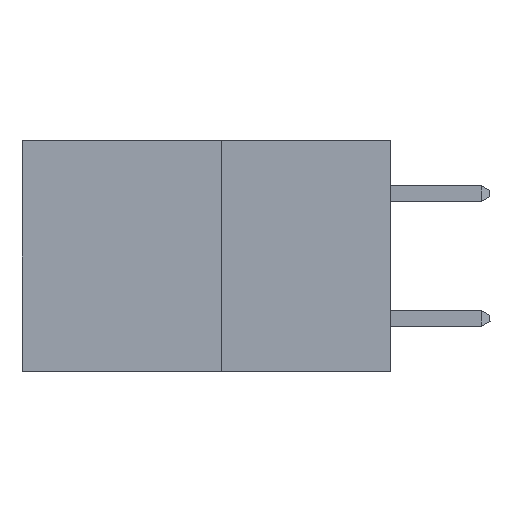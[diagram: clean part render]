
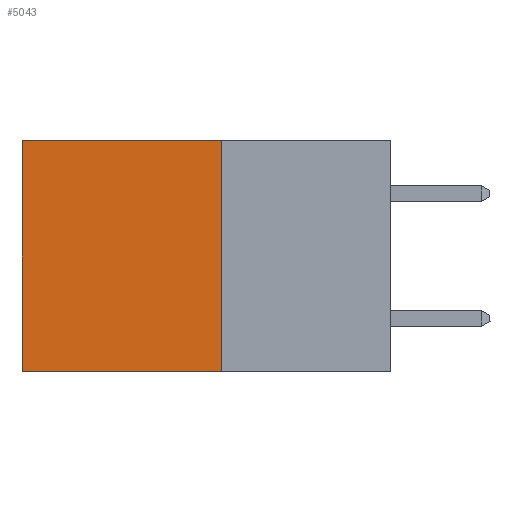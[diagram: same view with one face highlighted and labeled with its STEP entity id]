
A CAD part, left-side view. The second image highlights one B-rep face of the part: STEP entity #5043.
In plain terms, the highlighted planar face has unit normal (-1, 0, 0).
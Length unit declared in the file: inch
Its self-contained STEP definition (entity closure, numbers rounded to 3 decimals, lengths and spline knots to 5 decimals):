
#321 = AXIS2_PLACEMENT_3D ( 'NONE', #8548, #8375, #8352 ) ;
#361 = CARTESIAN_POINT ( 'NONE',  ( 0.277, 0.27, 0. ) ) ;
#3229 = DIRECTION ( 'NONE',  ( 0., 0., -1. ) ) ;
#4635 = VECTOR ( 'NONE', #23916, 39.37008 ) ;
#4870 = EDGE_CURVE ( 'NONE', #6382, #26060, #16829, .T. ) ;
#5043 = ADVANCED_FACE ( 'NONE', ( #12200 ), #8819, .F. ) ;
#5691 = CARTESIAN_POINT ( 'NONE',  ( 0.277, 0.27, 0. ) ) ;
#6382 = VERTEX_POINT ( 'NONE', #19928 ) ;
#6385 = CARTESIAN_POINT ( 'NONE',  ( 0.277, 0.59, 0. ) ) ;
#7436 = ORIENTED_EDGE ( 'NONE', *, *, #4870, .F. ) ;
#7509 = EDGE_CURVE ( 'NONE', #14707, #26060, #19439, .T. ) ;
#7871 = VERTEX_POINT ( 'NONE', #5691 ) ;
#8352 = DIRECTION ( 'NONE',  ( 0., 0., -1. ) ) ;
#8375 = DIRECTION ( 'NONE',  ( 1., 0., 0. ) ) ;
#8548 = CARTESIAN_POINT ( 'NONE',  ( 0.277, 0.27, -0.37 ) ) ;
#8819 = PLANE ( 'NONE',  #321 ) ;
#9080 = DIRECTION ( 'NONE',  ( 0., 0., -1. ) ) ;
#9460 = LINE ( 'NONE', #16090, #26317 ) ;
#11034 = ORIENTED_EDGE ( 'NONE', *, *, #15144, .F. ) ;
#11118 = LINE ( 'NONE', #361, #4635 ) ;
#11879 = VECTOR ( 'NONE', #12729, 39.37008 ) ;
#12200 = FACE_OUTER_BOUND ( 'NONE', #14894, .T. ) ;
#12729 = DIRECTION ( 'NONE',  ( 0., 1., 0. ) ) ;
#12757 = CARTESIAN_POINT ( 'NONE',  ( 0.277, 0.27, -0.37 ) ) ;
#13792 = VECTOR ( 'NONE', #9080, 39.37008 ) ;
#14707 = VERTEX_POINT ( 'NONE', #6385 ) ;
#14894 = EDGE_LOOP ( 'NONE', ( #15202, #7436, #11034, #25465 ) ) ;
#15144 = EDGE_CURVE ( 'NONE', #7871, #6382, #9460, .T. ) ;
#15202 = ORIENTED_EDGE ( 'NONE', *, *, #7509, .T. ) ;
#16090 = CARTESIAN_POINT ( 'NONE',  ( 0.277, 0.27, -0.37 ) ) ;
#16829 = LINE ( 'NONE', #12757, #11879 ) ;
#18511 = CARTESIAN_POINT ( 'NONE',  ( 0.277, 0.59, -0.37 ) ) ;
#19439 = LINE ( 'NONE', #19612, #13792 ) ;
#19612 = CARTESIAN_POINT ( 'NONE',  ( 0.277, 0.59, -0.37 ) ) ;
#19928 = CARTESIAN_POINT ( 'NONE',  ( 0.277, 0.27, -0.37 ) ) ;
#23916 = DIRECTION ( 'NONE',  ( 0., 1., 0. ) ) ;
#25465 = ORIENTED_EDGE ( 'NONE', *, *, #26993, .T. ) ;
#26060 = VERTEX_POINT ( 'NONE', #18511 ) ;
#26317 = VECTOR ( 'NONE', #3229, 39.37008 ) ;
#26993 = EDGE_CURVE ( 'NONE', #7871, #14707, #11118, .T. ) ;
